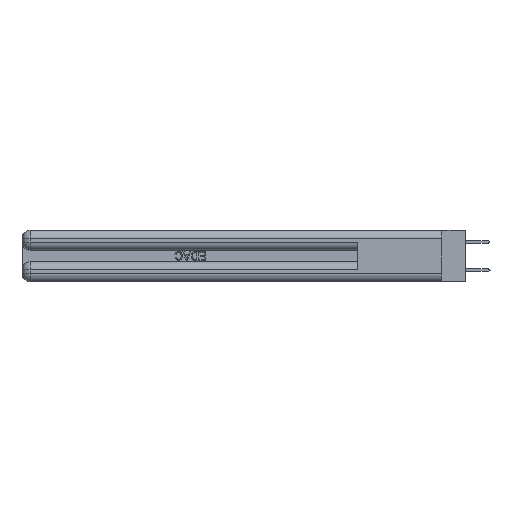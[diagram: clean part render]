
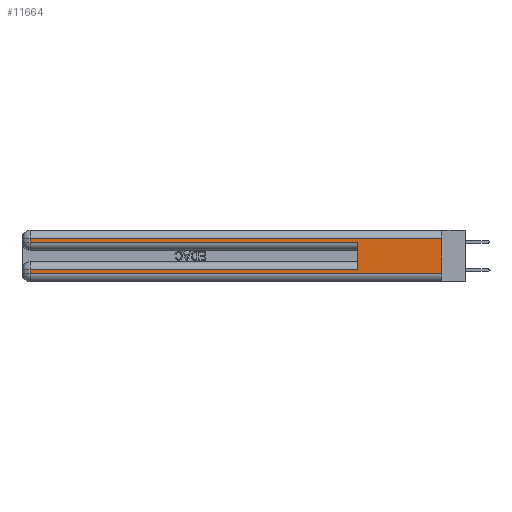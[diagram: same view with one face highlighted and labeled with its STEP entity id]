
A CAD part, left-side view. The second image highlights one B-rep face of the part: STEP entity #11664.
In plain terms, the highlighted planar face has unit normal (-1, 0, 0).
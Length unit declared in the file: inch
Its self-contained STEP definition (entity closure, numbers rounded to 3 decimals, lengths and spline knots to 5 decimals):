
#88 = EDGE_CURVE ( 'NONE', #1104, #5834, #2458, .T. ) ;
#465 = DIRECTION ( 'NONE',  ( 0., 0., -1. ) ) ;
#1104 = VERTEX_POINT ( 'NONE', #31168 ) ;
#1492 = CARTESIAN_POINT ( 'NONE',  ( 0., 0.6, 0.085 ) ) ;
#1691 = CARTESIAN_POINT ( 'NONE',  ( 0., 0., 0.31 ) ) ;
#2458 = LINE ( 'NONE', #22563, #21599 ) ;
#3326 = VERTEX_POINT ( 'NONE', #1492 ) ;
#4543 = DIRECTION ( 'NONE',  ( 0., -1., 0. ) ) ;
#5834 = VERTEX_POINT ( 'NONE', #42696 ) ;
#7466 = CARTESIAN_POINT ( 'NONE',  ( 0., 2.94, 0.285 ) ) ;
#7553 = VERTEX_POINT ( 'NONE', #23895 ) ;
#7710 = CARTESIAN_POINT ( 'NONE',  ( 0., 0., 0.31 ) ) ;
#8331 = ORIENTED_EDGE ( 'NONE', *, *, #9818, .T. ) ;
#9210 = FACE_OUTER_BOUND ( 'NONE', #14491, .T. ) ;
#9818 = EDGE_CURVE ( 'NONE', #40174, #28210, #39301, .T. ) ;
#10397 = VECTOR ( 'NONE', #41088, 39.37008 ) ;
#10974 = CARTESIAN_POINT ( 'NONE',  ( 0., 2.94, 0.37 ) ) ;
#11150 = LINE ( 'NONE', #44007, #44036 ) ;
#11569 = EDGE_CURVE ( 'NONE', #3326, #40704, #36998, .T. ) ;
#11664 = ADVANCED_FACE ( 'NONE', ( #9210 ), #31468, .F. ) ;
#12220 = VECTOR ( 'NONE', #30643, 39.37008 ) ;
#14491 = EDGE_LOOP ( 'NONE', ( #43504, #8331, #20383, #45026, #26639, #29354, #37857, #28776 ) ) ;
#14988 = DIRECTION ( 'NONE',  ( 1., 0., 0. ) ) ;
#15077 = DIRECTION ( 'NONE',  ( 0., 0., -1. ) ) ;
#15162 = DIRECTION ( 'NONE',  ( 0., 0., 1. ) ) ;
#16068 = EDGE_CURVE ( 'NONE', #3326, #7553, #11150, .T. ) ;
#16958 = CARTESIAN_POINT ( 'NONE',  ( 0., 2.94, 0.31 ) ) ;
#18870 = VECTOR ( 'NONE', #15077, 39.37008 ) ;
#19508 = CARTESIAN_POINT ( 'NONE',  ( 0., 0., 0.37 ) ) ;
#20383 = ORIENTED_EDGE ( 'NONE', *, *, #25391, .T. ) ;
#21469 = CARTESIAN_POINT ( 'NONE',  ( 0., 0., 0.37 ) ) ;
#21599 = VECTOR ( 'NONE', #4543, 39.37008 ) ;
#21746 = CARTESIAN_POINT ( 'NONE',  ( 0., 0., 0.085 ) ) ;
#21834 = CARTESIAN_POINT ( 'NONE',  ( 0., 0., 0.285 ) ) ;
#22563 = CARTESIAN_POINT ( 'NONE',  ( 0., 0., 0.06 ) ) ;
#23015 = DIRECTION ( 'NONE',  ( 0., 1., 0. ) ) ;
#23671 = LINE ( 'NONE', #21834, #34453 ) ;
#23895 = CARTESIAN_POINT ( 'NONE',  ( 0., 0.6, 0.285 ) ) ;
#25391 = EDGE_CURVE ( 'NONE', #28210, #32186, #45741, .T. ) ;
#25628 = CARTESIAN_POINT ( 'NONE',  ( 0., 2.94, 0.37 ) ) ;
#26159 = EDGE_CURVE ( 'NONE', #40174, #5834, #28701, .T. ) ;
#26204 = CARTESIAN_POINT ( 'NONE',  ( 0., 2.94, 0.085 ) ) ;
#26639 = ORIENTED_EDGE ( 'NONE', *, *, #16068, .F. ) ;
#27850 = EDGE_CURVE ( 'NONE', #40704, #1104, #28533, .T. ) ;
#28210 = VERTEX_POINT ( 'NONE', #16958 ) ;
#28533 = LINE ( 'NONE', #10974, #18870 ) ;
#28701 = LINE ( 'NONE', #19508, #12220 ) ;
#28776 = ORIENTED_EDGE ( 'NONE', *, *, #88, .T. ) ;
#29354 = ORIENTED_EDGE ( 'NONE', *, *, #11569, .T. ) ;
#30643 = DIRECTION ( 'NONE',  ( 0., 0., -1. ) ) ;
#31168 = CARTESIAN_POINT ( 'NONE',  ( 0., 2.94, 0.06 ) ) ;
#31468 = PLANE ( 'NONE',  #32529 ) ;
#32186 = VERTEX_POINT ( 'NONE', #7466 ) ;
#32529 = AXIS2_PLACEMENT_3D ( 'NONE', #21469, #14988, #465 ) ;
#34442 = VECTOR ( 'NONE', #44955, 39.37008 ) ;
#34453 = VECTOR ( 'NONE', #43580, 39.37008 ) ;
#36998 = LINE ( 'NONE', #21746, #41012 ) ;
#37857 = ORIENTED_EDGE ( 'NONE', *, *, #27850, .T. ) ;
#39301 = LINE ( 'NONE', #1691, #10397 ) ;
#40174 = VERTEX_POINT ( 'NONE', #7710 ) ;
#40704 = VERTEX_POINT ( 'NONE', #26204 ) ;
#41012 = VECTOR ( 'NONE', #23015, 39.37008 ) ;
#41088 = DIRECTION ( 'NONE',  ( 0., 1., 0. ) ) ;
#42696 = CARTESIAN_POINT ( 'NONE',  ( 0., 0., 0.06 ) ) ;
#43504 = ORIENTED_EDGE ( 'NONE', *, *, #26159, .F. ) ;
#43580 = DIRECTION ( 'NONE',  ( 0., -1., 0. ) ) ;
#44007 = CARTESIAN_POINT ( 'NONE',  ( 0., 0.6, 0.145 ) ) ;
#44036 = VECTOR ( 'NONE', #15162, 39.37008 ) ;
#44285 = EDGE_CURVE ( 'NONE', #32186, #7553, #23671, .T. ) ;
#44955 = DIRECTION ( 'NONE',  ( 0., 0., -1. ) ) ;
#45026 = ORIENTED_EDGE ( 'NONE', *, *, #44285, .T. ) ;
#45741 = LINE ( 'NONE', #25628, #34442 ) ;
